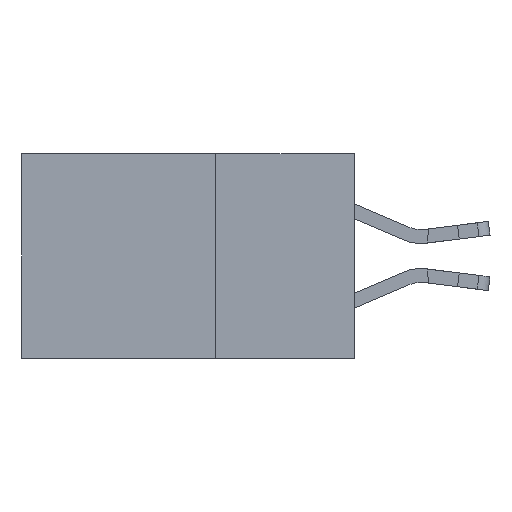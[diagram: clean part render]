
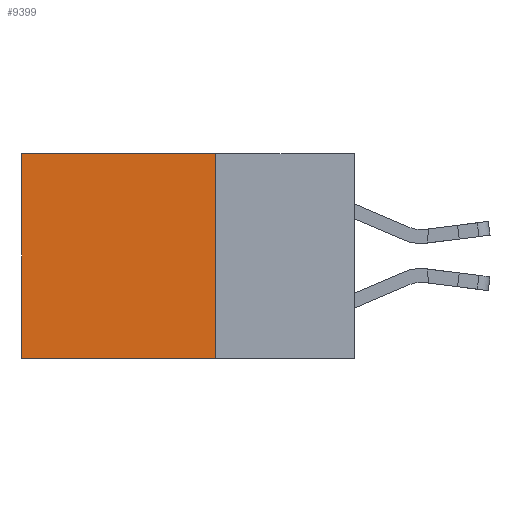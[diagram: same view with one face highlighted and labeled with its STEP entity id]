
A CAD part, left-side view. The second image highlights one B-rep face of the part: STEP entity #9399.
In plain terms, the highlighted planar face has unit normal (-1, 0, 0).
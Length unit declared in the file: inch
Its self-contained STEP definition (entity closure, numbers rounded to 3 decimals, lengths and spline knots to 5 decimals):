
#680 = EDGE_CURVE ( 'NONE', #13854, #2780, #15623, .T. ) ;
#820 = VECTOR ( 'NONE', #5442, 39.37008 ) ;
#1014 = LINE ( 'NONE', #17324, #4489 ) ;
#1114 = CARTESIAN_POINT ( 'NONE',  ( 0.298, 0.25, 0. ) ) ;
#1869 = EDGE_CURVE ( 'NONE', #11087, #2780, #1014, .T. ) ;
#2076 = ORIENTED_EDGE ( 'NONE', *, *, #16021, .T. ) ;
#2494 = DIRECTION ( 'NONE',  ( 0., 1., 0. ) ) ;
#2780 = VERTEX_POINT ( 'NONE', #2924 ) ;
#2924 = CARTESIAN_POINT ( 'NONE',  ( 0.298, 0.6, -0.37 ) ) ;
#3338 = CARTESIAN_POINT ( 'NONE',  ( 0.298, 0.6, 0. ) ) ;
#3680 = ORIENTED_EDGE ( 'NONE', *, *, #1869, .F. ) ;
#4489 = VECTOR ( 'NONE', #17980, 39.37008 ) ;
#5442 = DIRECTION ( 'NONE',  ( 0., 0., -1. ) ) ;
#6173 = EDGE_LOOP ( 'NONE', ( #9907, #3680, #11556, #2076 ) ) ;
#6688 = PLANE ( 'NONE',  #8833 ) ;
#6863 = CARTESIAN_POINT ( 'NONE',  ( 0.298, 0.25, 0. ) ) ;
#8088 = CARTESIAN_POINT ( 'NONE',  ( 0.298, 0.25, 0. ) ) ;
#8316 = VERTEX_POINT ( 'NONE', #1114 ) ;
#8833 = AXIS2_PLACEMENT_3D ( 'NONE', #16565, #18005, #9511 ) ;
#9144 = FACE_OUTER_BOUND ( 'NONE', #6173, .T. ) ;
#9399 = ADVANCED_FACE ( 'NONE', ( #9144 ), #6688, .F. ) ;
#9439 = LINE ( 'NONE', #6863, #16532 ) ;
#9511 = DIRECTION ( 'NONE',  ( 0., 0., -1. ) ) ;
#9907 = ORIENTED_EDGE ( 'NONE', *, *, #680, .T. ) ;
#11087 = VERTEX_POINT ( 'NONE', #12514 ) ;
#11556 = ORIENTED_EDGE ( 'NONE', *, *, #17707, .F. ) ;
#12514 = CARTESIAN_POINT ( 'NONE',  ( 0.298, 0.25, -0.37 ) ) ;
#12702 = VECTOR ( 'NONE', #16643, 39.37008 ) ;
#13854 = VERTEX_POINT ( 'NONE', #15862 ) ;
#15623 = LINE ( 'NONE', #3338, #820 ) ;
#15862 = CARTESIAN_POINT ( 'NONE',  ( 0.298, 0.6, 0. ) ) ;
#16021 = EDGE_CURVE ( 'NONE', #8316, #13854, #9439, .T. ) ;
#16463 = LINE ( 'NONE', #8088, #12702 ) ;
#16532 = VECTOR ( 'NONE', #2494, 39.37008 ) ;
#16565 = CARTESIAN_POINT ( 'NONE',  ( 0.298, 0.25, 0. ) ) ;
#16643 = DIRECTION ( 'NONE',  ( 0., 0., -1. ) ) ;
#17324 = CARTESIAN_POINT ( 'NONE',  ( 0.298, 0.25, -0.37 ) ) ;
#17707 = EDGE_CURVE ( 'NONE', #8316, #11087, #16463, .T. ) ;
#17980 = DIRECTION ( 'NONE',  ( 0., 1., 0. ) ) ;
#18005 = DIRECTION ( 'NONE',  ( 1., 0., 0. ) ) ;
